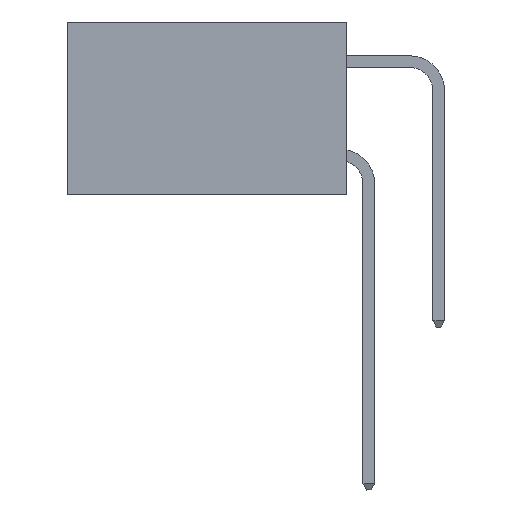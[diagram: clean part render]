
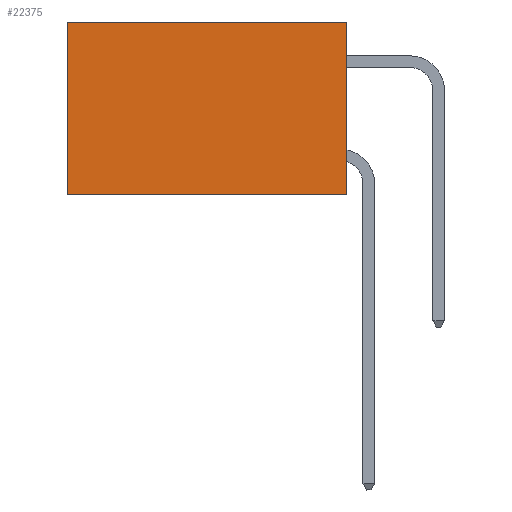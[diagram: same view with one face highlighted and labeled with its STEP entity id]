
A CAD part, left-side view. The second image highlights one B-rep face of the part: STEP entity #22375.
In plain terms, the highlighted planar face has unit normal (-1, 0, 0).
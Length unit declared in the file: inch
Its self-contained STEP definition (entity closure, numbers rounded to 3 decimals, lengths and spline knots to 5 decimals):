
#336 = ORIENTED_EDGE ( 'NONE', *, *, #28065, .F. ) ;
#1530 = DIRECTION ( 'NONE',  ( 0., 0., -1. ) ) ;
#2749 = CARTESIAN_POINT ( 'NONE',  ( 0.2875, 0., -0.37 ) ) ;
#2930 = VECTOR ( 'NONE', #6415, 39.37008 ) ;
#4064 = LINE ( 'NONE', #22973, #36549 ) ;
#6415 = DIRECTION ( 'NONE',  ( 0., 0., -1. ) ) ;
#6484 = CARTESIAN_POINT ( 'NONE',  ( 0.2875, 0., 0. ) ) ;
#8860 = VECTOR ( 'NONE', #17018, 39.37008 ) ;
#8884 = VERTEX_POINT ( 'NONE', #2749 ) ;
#10714 = LINE ( 'NONE', #23175, #2930 ) ;
#11121 = VERTEX_POINT ( 'NONE', #21442 ) ;
#13327 = DIRECTION ( 'NONE',  ( 0., 1., 0. ) ) ;
#16638 = VERTEX_POINT ( 'NONE', #21549 ) ;
#17018 = DIRECTION ( 'NONE',  ( 0., 0., -1. ) ) ;
#17297 = CARTESIAN_POINT ( 'NONE',  ( 0.2875, 0.6, 0. ) ) ;
#21146 = EDGE_CURVE ( 'NONE', #16638, #8884, #10714, .T. ) ;
#21442 = CARTESIAN_POINT ( 'NONE',  ( 0.2875, 0.6, -0.37 ) ) ;
#21549 = CARTESIAN_POINT ( 'NONE',  ( 0.2875, 0., 0. ) ) ;
#22375 = ADVANCED_FACE ( 'NONE', ( #25617 ), #31731, .F. ) ;
#22973 = CARTESIAN_POINT ( 'NONE',  ( 0.2875, 0., -0.37 ) ) ;
#23175 = CARTESIAN_POINT ( 'NONE',  ( 0.2875, 0., 0. ) ) ;
#23460 = EDGE_CURVE ( 'NONE', #16638, #30824, #34770, .T. ) ;
#25256 = ORIENTED_EDGE ( 'NONE', *, *, #21146, .F. ) ;
#25617 = FACE_OUTER_BOUND ( 'NONE', #32396, .T. ) ;
#26036 = VECTOR ( 'NONE', #32868, 39.37008 ) ;
#27243 = DIRECTION ( 'NONE',  ( 1., 0., 0. ) ) ;
#28065 = EDGE_CURVE ( 'NONE', #8884, #11121, #4064, .T. ) ;
#29494 = LINE ( 'NONE', #17297, #8860 ) ;
#30660 = AXIS2_PLACEMENT_3D ( 'NONE', #32014, #27243, #1530 ) ;
#30824 = VERTEX_POINT ( 'NONE', #39400 ) ;
#31731 = PLANE ( 'NONE',  #30660 ) ;
#32014 = CARTESIAN_POINT ( 'NONE',  ( 0.2875, 0., 0. ) ) ;
#32396 = EDGE_LOOP ( 'NONE', ( #41120, #336, #25256, #33903 ) ) ;
#32868 = DIRECTION ( 'NONE',  ( 0., 1., 0. ) ) ;
#33903 = ORIENTED_EDGE ( 'NONE', *, *, #23460, .T. ) ;
#34384 = EDGE_CURVE ( 'NONE', #30824, #11121, #29494, .T. ) ;
#34770 = LINE ( 'NONE', #6484, #26036 ) ;
#36549 = VECTOR ( 'NONE', #13327, 39.37008 ) ;
#39400 = CARTESIAN_POINT ( 'NONE',  ( 0.2875, 0.6, 0. ) ) ;
#41120 = ORIENTED_EDGE ( 'NONE', *, *, #34384, .T. ) ;
